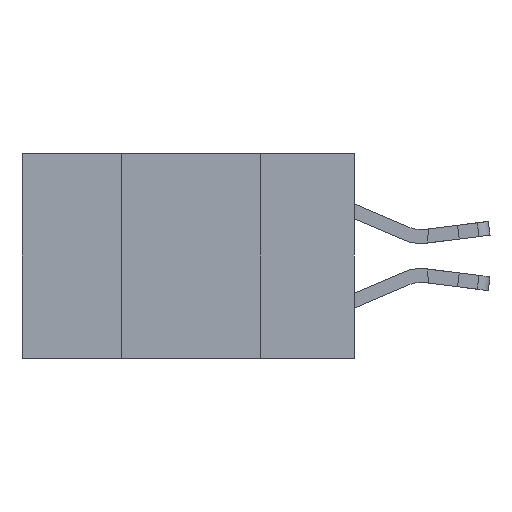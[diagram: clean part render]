
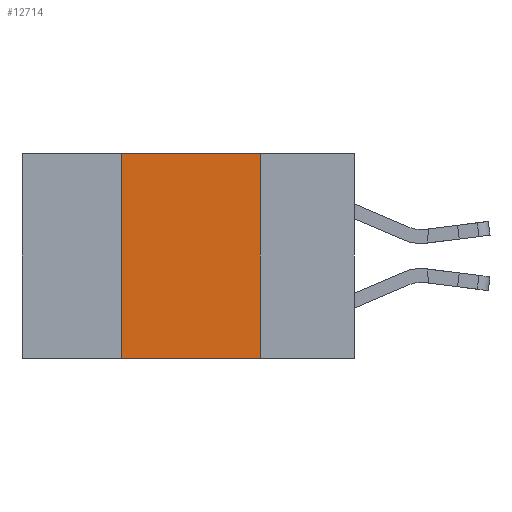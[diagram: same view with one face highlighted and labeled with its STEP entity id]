
A CAD part, left-side view. The second image highlights one B-rep face of the part: STEP entity #12714.
In plain terms, the highlighted planar face has unit normal (-1, 0, 0).
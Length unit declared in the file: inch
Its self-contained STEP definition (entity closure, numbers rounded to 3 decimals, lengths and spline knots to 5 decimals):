
#155 = DIRECTION ( 'NONE',  ( 0., 0., 1. ) ) ;
#236 = LINE ( 'NONE', #15346, #10947 ) ;
#1011 = CARTESIAN_POINT ( 'NONE',  ( 0., 0.42, -0.37 ) ) ;
#1249 = CARTESIAN_POINT ( 'NONE',  ( 0., 0.6, 0. ) ) ;
#1467 = VERTEX_POINT ( 'NONE', #8790 ) ;
#1740 = CARTESIAN_POINT ( 'NONE',  ( 0., 0.6, 0. ) ) ;
#1887 = VECTOR ( 'NONE', #2703, 39.37008 ) ;
#2023 = EDGE_CURVE ( 'NONE', #10856, #1467, #236, .T. ) ;
#2703 = DIRECTION ( 'NONE',  ( 0., -1., 0. ) ) ;
#3177 = DIRECTION ( 'NONE',  ( 1., 0., 0. ) ) ;
#3642 = CARTESIAN_POINT ( 'NONE',  ( 0., 0.42, 0. ) ) ;
#5542 = ORIENTED_EDGE ( 'NONE', *, *, #2023, .T. ) ;
#5948 = CARTESIAN_POINT ( 'NONE',  ( 0., 0.42, 0. ) ) ;
#6064 = PLANE ( 'NONE',  #7462 ) ;
#6617 = VECTOR ( 'NONE', #155, 39.37008 ) ;
#6686 = LINE ( 'NONE', #1249, #1887 ) ;
#7073 = LINE ( 'NONE', #5948, #6617 ) ;
#7462 = AXIS2_PLACEMENT_3D ( 'NONE', #1740, #3177, #13342 ) ;
#7941 = CARTESIAN_POINT ( 'NONE',  ( 0., 0.17, 0. ) ) ;
#8172 = DIRECTION ( 'NONE',  ( 0., -1., 0. ) ) ;
#8502 = LINE ( 'NONE', #17108, #15714 ) ;
#8510 = DIRECTION ( 'NONE',  ( 0., 0., -1. ) ) ;
#8790 = CARTESIAN_POINT ( 'NONE',  ( 0., 0.17, -0.37 ) ) ;
#10856 = VERTEX_POINT ( 'NONE', #1011 ) ;
#10936 = EDGE_CURVE ( 'NONE', #14126, #1467, #8502, .T. ) ;
#10947 = VECTOR ( 'NONE', #8172, 39.37008 ) ;
#11486 = EDGE_CURVE ( 'NONE', #16418, #14126, #6686, .T. ) ;
#12087 = FACE_OUTER_BOUND ( 'NONE', #14698, .T. ) ;
#12714 = ADVANCED_FACE ( 'NONE', ( #12087 ), #6064, .F. ) ;
#13342 = DIRECTION ( 'NONE',  ( 0., 0., -1. ) ) ;
#13906 = EDGE_CURVE ( 'NONE', #10856, #16418, #7073, .T. ) ;
#14126 = VERTEX_POINT ( 'NONE', #7941 ) ;
#14144 = ORIENTED_EDGE ( 'NONE', *, *, #13906, .F. ) ;
#14698 = EDGE_LOOP ( 'NONE', ( #18241, #15777, #14144, #5542 ) ) ;
#15346 = CARTESIAN_POINT ( 'NONE',  ( 0., 0.6, -0.37 ) ) ;
#15714 = VECTOR ( 'NONE', #8510, 39.37008 ) ;
#15777 = ORIENTED_EDGE ( 'NONE', *, *, #11486, .F. ) ;
#16418 = VERTEX_POINT ( 'NONE', #3642 ) ;
#17108 = CARTESIAN_POINT ( 'NONE',  ( 0., 0.17, 0. ) ) ;
#18241 = ORIENTED_EDGE ( 'NONE', *, *, #10936, .F. ) ;
